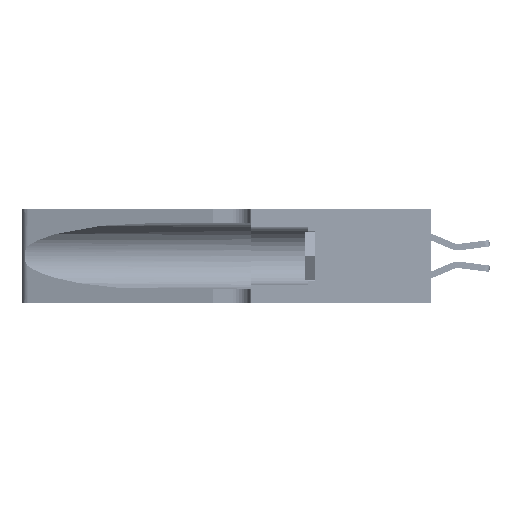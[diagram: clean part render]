
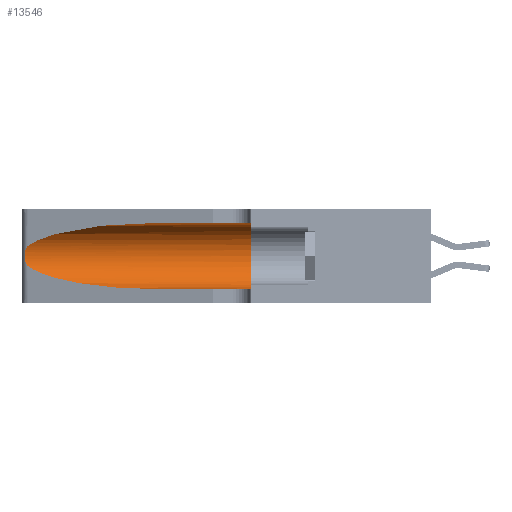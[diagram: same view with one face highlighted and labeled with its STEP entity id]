
A CAD part, left-side view. The second image highlights one B-rep face of the part: STEP entity #13546.
In plain terms, the highlighted cylindrical face has radius 3.308 mm (diameter 6.617 mm), a partial arc.
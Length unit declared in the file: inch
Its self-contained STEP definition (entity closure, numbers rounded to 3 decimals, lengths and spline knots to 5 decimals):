
#413 = EDGE_CURVE ( 'NONE', #27976, #28866, #12901, .T. ) ;
#657 = CARTESIAN_POINT ( 'NONE',  ( 0.25487, 1.22718, 0.22369 ) ) ;
#676 = CARTESIAN_POINT ( 'NONE',  ( 0.25487, 1.22718, 0.14631 ) ) ;
#1180 = EDGE_LOOP ( 'NONE', ( #4326, #18552, #36290, #25683, #10153, #8656 ) ) ;
#2989 = CARTESIAN_POINT ( 'NONE',  ( 0.25789, 1.23486, 0.15765 ) ) ;
#3324 = CARTESIAN_POINT ( 'NONE',  ( 0.1305, 0.72297, 0.31525 ) ) ;
#4326 = ORIENTED_EDGE ( 'NONE', *, *, #34810, .T. ) ;
#4520 = CARTESIAN_POINT ( 'NONE',  ( 0.1305, 1.61858, 0.185 ) ) ;
#5418 = CARTESIAN_POINT ( 'NONE',  ( 0.25487, 1.22718, 0.14631 ) ) ;
#6001 = CARTESIAN_POINT ( 'NONE',  ( 0.25639, 1.23186, 0.15144 ) ) ;
#6629 = FACE_OUTER_BOUND ( 'NONE', #1180, .T. ) ;
#7662 = DIRECTION ( 'NONE',  ( 0., 0., -1. ) ) ;
#8656 = ORIENTED_EDGE ( 'NONE', *, *, #31732, .F. ) ;
#9357 = CARTESIAN_POINT ( 'NONE',  ( 0.1305, 0.35, 0.05475 ) ) ;
#9428 = CARTESIAN_POINT ( 'NONE',  ( 0.1305, 0.72297, 0.05475 ) ) ;
#10153 = ORIENTED_EDGE ( 'NONE', *, *, #18993, .F. ) ;
#11510 = CARTESIAN_POINT ( 'NONE',  ( 0.2373, 1.15595, 0.08982 ) ) ;
#12257 = CARTESIAN_POINT ( 'NONE',  ( 0.25639, 1.23184, 0.21858 ) ) ;
#12901 =( BOUNDED_CURVE ( )  B_SPLINE_CURVE ( 3, ( #5418, #11510, #14396, #23884 ),
 .UNSPECIFIED., .F., .T. ) 
 B_SPLINE_CURVE_WITH_KNOTS ( ( 4, 4 ),
 ( 3.44316, 4.71239 ),
 .UNSPECIFIED. ) 
 CURVE ( )  GEOMETRIC_REPRESENTATION_ITEM ( )  RATIONAL_B_SPLINE_CURVE ( ( 1., 0.87, 0.87, 1. ) ) 
 REPRESENTATION_ITEM ( '' )  );
#13546 = ADVANCED_FACE ( 'NONE', ( #6629 ), #17520, .F. ) ;
#14135 = CARTESIAN_POINT ( 'NONE',  ( 0.2373, 1.15595, 0.28018 ) ) ;
#14396 = CARTESIAN_POINT ( 'NONE',  ( 0.18966, 0.96281, 0.05475 ) ) ;
#15088 = CARTESIAN_POINT ( 'NONE',  ( 0.1305, 0.35, 0.31525 ) ) ;
#15546 = CARTESIAN_POINT ( 'NONE',  ( 0.25487, 1.22718, 0.22369 ) ) ;
#17520 = CYLINDRICAL_SURFACE ( 'NONE', #22769, 0.13025 ) ;
#17692 = LINE ( 'NONE', #38981, #25070 ) ;
#18552 = ORIENTED_EDGE ( 'NONE', *, *, #25628, .T. ) ;
#18583 = CARTESIAN_POINT ( 'NONE',  ( 0.25854, 1.2359, 0.20912 ) ) ;
#18983 = CARTESIAN_POINT ( 'NONE',  ( 0.25555, 1.22994, 0.2215 ) ) ;
#18993 = EDGE_CURVE ( 'NONE', #36912, #40658, #19078, .T. ) ;
#19078 = CIRCLE ( 'NONE', #22364, 0.13025 ) ;
#20717 = CARTESIAN_POINT ( 'NONE',  ( 0.25487, 1.22718, 0.22369 ) ) ;
#21735 = CARTESIAN_POINT ( 'NONE',  ( 0.25555, 1.22993, 0.14849 ) ) ;
#21969 = B_SPLINE_CURVE_WITH_KNOTS ( 'NONE', 3,
 ( #15546, #18983, #12257, #25431, #18583, #31095, #34577, #31371, #27935, #31233, #2989, #6001, #21735, #30800 ),
 .UNSPECIFIED., .F., .F.,
 ( 4, 2, 2, 2, 2, 2, 4 ),
 ( 0., 0.00027, 0.00053, 0.00107, 0.0016, 0.00187, 0.00214 ),
 .UNSPECIFIED. ) ;
#22364 = AXIS2_PLACEMENT_3D ( 'NONE', #33638, #40790, #22745 ) ;
#22745 = DIRECTION ( 'NONE',  ( 0., 0., 1. ) ) ;
#22769 = AXIS2_PLACEMENT_3D ( 'NONE', #4520, #26559, #7662 ) ;
#22898 = CARTESIAN_POINT ( 'NONE',  ( 0.18966, 0.96281, 0.31525 ) ) ;
#23884 = CARTESIAN_POINT ( 'NONE',  ( 0.1305, 0.72297, 0.05475 ) ) ;
#24055 = DIRECTION ( 'NONE',  ( 0., -1., 0. ) ) ;
#25070 = VECTOR ( 'NONE', #24055, 39.37008 ) ;
#25431 = CARTESIAN_POINT ( 'NONE',  ( 0.25787, 1.23484, 0.2124 ) ) ;
#25628 = EDGE_CURVE ( 'NONE', #36572, #27976, #21969, .T. ) ;
#25683 = ORIENTED_EDGE ( 'NONE', *, *, #28616, .T. ) ;
#26559 = DIRECTION ( 'NONE',  ( 0., -1., 0. ) ) ;
#27595 = CARTESIAN_POINT ( 'NONE',  ( 0.1305, 1.61858, 0.31525 ) ) ;
#27935 = CARTESIAN_POINT ( 'NONE',  ( 0.26017, 1.23833, 0.17102 ) ) ;
#27976 = VERTEX_POINT ( 'NONE', #676 ) ;
#28616 = EDGE_CURVE ( 'NONE', #28866, #40658, #17692, .T. ) ;
#28866 = VERTEX_POINT ( 'NONE', #9428 ) ;
#30800 = CARTESIAN_POINT ( 'NONE',  ( 0.25487, 1.22718, 0.14631 ) ) ;
#31095 = CARTESIAN_POINT ( 'NONE',  ( 0.26018, 1.23835, 0.19895 ) ) ;
#31233 = CARTESIAN_POINT ( 'NONE',  ( 0.25856, 1.23593, 0.16098 ) ) ;
#31371 = CARTESIAN_POINT ( 'NONE',  ( 0.26075, 1.23896, 0.178 ) ) ;
#31732 = EDGE_CURVE ( 'NONE', #31960, #36912, #32657, .T. ) ;
#31960 = VERTEX_POINT ( 'NONE', #3324 ) ;
#32245 =( BOUNDED_CURVE ( )  B_SPLINE_CURVE ( 3, ( #38516, #22898, #14135, #20717 ),
 .UNSPECIFIED., .F., .F. ) 
 B_SPLINE_CURVE_WITH_KNOTS ( ( 4, 4 ),
 ( 1.5708, 2.84003 ),
 .UNSPECIFIED. ) 
 CURVE ( )  GEOMETRIC_REPRESENTATION_ITEM ( )  RATIONAL_B_SPLINE_CURVE ( ( 1., 0.87, 0.87, 1. ) ) 
 REPRESENTATION_ITEM ( '' )  );
#32657 = LINE ( 'NONE', #27595, #40525 ) ;
#33638 = CARTESIAN_POINT ( 'NONE',  ( 0.1305, 0.35, 0.185 ) ) ;
#34577 = CARTESIAN_POINT ( 'NONE',  ( 0.26075, 1.23896, 0.19203 ) ) ;
#34810 = EDGE_CURVE ( 'NONE', #31960, #36572, #32245, .T. ) ;
#36290 = ORIENTED_EDGE ( 'NONE', *, *, #413, .T. ) ;
#36572 = VERTEX_POINT ( 'NONE', #657 ) ;
#36590 = DIRECTION ( 'NONE',  ( 0., -1., 0. ) ) ;
#36912 = VERTEX_POINT ( 'NONE', #15088 ) ;
#38516 = CARTESIAN_POINT ( 'NONE',  ( 0.1305, 0.72297, 0.31525 ) ) ;
#38981 = CARTESIAN_POINT ( 'NONE',  ( 0.1305, 1.61858, 0.05475 ) ) ;
#40525 = VECTOR ( 'NONE', #36590, 39.37008 ) ;
#40658 = VERTEX_POINT ( 'NONE', #9357 ) ;
#40790 = DIRECTION ( 'NONE',  ( 0., 1., 0. ) ) ;
